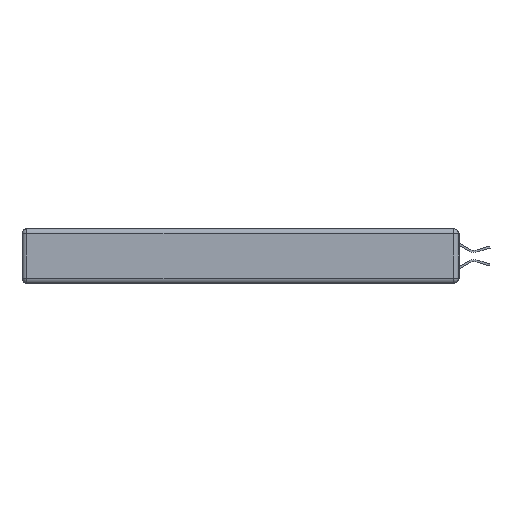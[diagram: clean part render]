
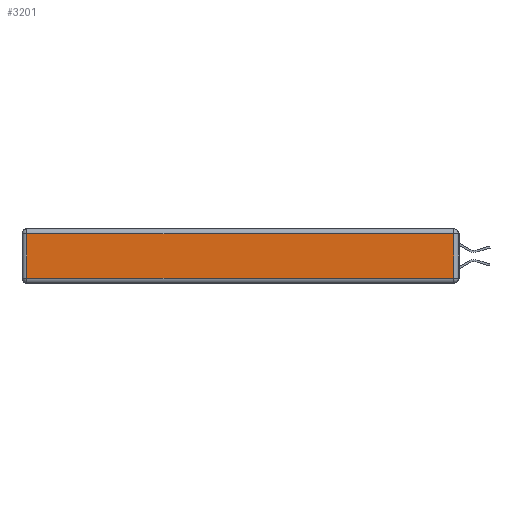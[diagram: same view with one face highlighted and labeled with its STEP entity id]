
A CAD part, left-side view. The second image highlights one B-rep face of the part: STEP entity #3201.
In plain terms, the highlighted planar face has unit normal (-1, 0, 0).
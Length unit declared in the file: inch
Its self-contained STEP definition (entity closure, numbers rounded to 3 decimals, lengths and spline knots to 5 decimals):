
#376 = CARTESIAN_POINT ( 'NONE',  ( 0., 0., -0.313 ) ) ;
#1247 = CARTESIAN_POINT ( 'NONE',  ( 0., 0.03, -0.343 ) ) ;
#2546 = LINE ( 'NONE', #9520, #16188 ) ;
#3201 = ADVANCED_FACE ( 'NONE', ( #18196 ), #7896, .T. ) ;
#4623 = DIRECTION ( 'NONE',  ( -1., 0., 0. ) ) ;
#4741 = EDGE_CURVE ( 'NONE', #19435, #8059, #2546, .T. ) ;
#4817 = DIRECTION ( 'NONE',  ( 0., 1., 0. ) ) ;
#6422 = CARTESIAN_POINT ( 'NONE',  ( 0., 2.72, -0.03 ) ) ;
#7019 = EDGE_CURVE ( 'NONE', #16721, #19435, #20120, .T. ) ;
#7056 = VECTOR ( 'NONE', #13257, 39.37008 ) ;
#7338 = DIRECTION ( 'NONE',  ( 0., -1., 0. ) ) ;
#7772 = CARTESIAN_POINT ( 'NONE',  ( 0., 0.03, -0.03 ) ) ;
#7896 = PLANE ( 'NONE',  #10359 ) ;
#8059 = VERTEX_POINT ( 'NONE', #6422 ) ;
#8296 = DIRECTION ( 'NONE',  ( 0., 0., -1. ) ) ;
#9520 = CARTESIAN_POINT ( 'NONE',  ( 0., 2.75, -0.03 ) ) ;
#9895 = ORIENTED_EDGE ( 'NONE', *, *, #10683, .T. ) ;
#10359 = AXIS2_PLACEMENT_3D ( 'NONE', #22382, #4623, #11854 ) ;
#10683 = EDGE_CURVE ( 'NONE', #8059, #18087, #13454, .T. ) ;
#11329 = CARTESIAN_POINT ( 'NONE',  ( 0., 2.72, -0.313 ) ) ;
#11482 = EDGE_CURVE ( 'NONE', #18087, #16721, #14777, .T. ) ;
#11535 = VECTOR ( 'NONE', #8296, 39.37008 ) ;
#11854 = DIRECTION ( 'NONE',  ( 0., 0., 1. ) ) ;
#12607 = CARTESIAN_POINT ( 'NONE',  ( 0., 0.03, -0.313 ) ) ;
#12645 = EDGE_LOOP ( 'NONE', ( #17869, #15725, #15343, #9895 ) ) ;
#13257 = DIRECTION ( 'NONE',  ( 0., 0., 1. ) ) ;
#13454 = LINE ( 'NONE', #22041, #11535 ) ;
#14777 = LINE ( 'NONE', #376, #16996 ) ;
#15343 = ORIENTED_EDGE ( 'NONE', *, *, #4741, .T. ) ;
#15725 = ORIENTED_EDGE ( 'NONE', *, *, #7019, .T. ) ;
#16188 = VECTOR ( 'NONE', #4817, 39.37008 ) ;
#16721 = VERTEX_POINT ( 'NONE', #12607 ) ;
#16996 = VECTOR ( 'NONE', #7338, 39.37008 ) ;
#17869 = ORIENTED_EDGE ( 'NONE', *, *, #11482, .T. ) ;
#18087 = VERTEX_POINT ( 'NONE', #11329 ) ;
#18196 = FACE_OUTER_BOUND ( 'NONE', #12645, .T. ) ;
#19435 = VERTEX_POINT ( 'NONE', #7772 ) ;
#20120 = LINE ( 'NONE', #1247, #7056 ) ;
#22041 = CARTESIAN_POINT ( 'NONE',  ( 0., 2.72, -0.343 ) ) ;
#22382 = CARTESIAN_POINT ( 'NONE',  ( 0., 0., -0.343 ) ) ;
